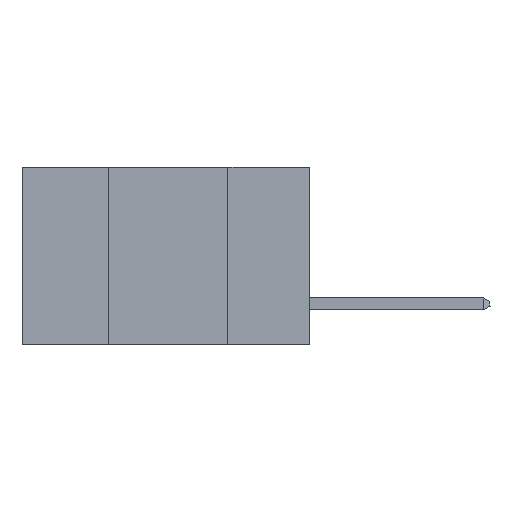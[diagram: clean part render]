
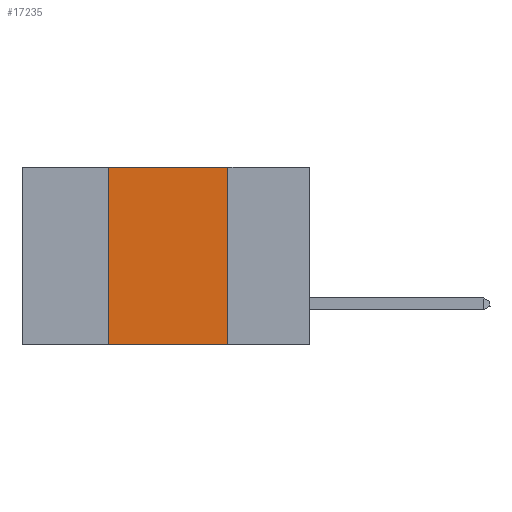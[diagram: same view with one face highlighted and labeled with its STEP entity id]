
A CAD part, left-side view. The second image highlights one B-rep face of the part: STEP entity #17235.
In plain terms, the highlighted planar face has unit normal (-1, 0, 0).
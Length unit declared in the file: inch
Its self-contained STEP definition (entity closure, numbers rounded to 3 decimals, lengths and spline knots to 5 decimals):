
#350 = FACE_OUTER_BOUND ( 'NONE', #6859, .T. ) ;
#2201 = CARTESIAN_POINT ( 'NONE',  ( 0., 0.42, 0. ) ) ;
#5978 = EDGE_CURVE ( 'NONE', #37490, #9699, #15782, .T. ) ;
#6859 = EDGE_LOOP ( 'NONE', ( #36666, #28218, #33068, #27287 ) ) ;
#7327 = LINE ( 'NONE', #34295, #31091 ) ;
#7467 = EDGE_CURVE ( 'NONE', #17618, #29254, #31325, .T. ) ;
#7757 = CARTESIAN_POINT ( 'NONE',  ( 0., 0.6, -0.37 ) ) ;
#9699 = VERTEX_POINT ( 'NONE', #17361 ) ;
#13880 = DIRECTION ( 'NONE',  ( 1., 0., 0. ) ) ;
#14411 = DIRECTION ( 'NONE',  ( 0., -1., 0. ) ) ;
#15782 = LINE ( 'NONE', #23435, #30913 ) ;
#17235 = ADVANCED_FACE ( 'NONE', ( #350 ), #18051, .F. ) ;
#17361 = CARTESIAN_POINT ( 'NONE',  ( 0., 0.17, -0.37 ) ) ;
#17618 = VERTEX_POINT ( 'NONE', #36976 ) ;
#17641 = CARTESIAN_POINT ( 'NONE',  ( 0., 0.42, 0. ) ) ;
#18051 = PLANE ( 'NONE',  #28806 ) ;
#19274 = EDGE_CURVE ( 'NONE', #29254, #37490, #7327, .T. ) ;
#20210 = CARTESIAN_POINT ( 'NONE',  ( 0., 0.6, 0. ) ) ;
#22496 = EDGE_CURVE ( 'NONE', #17618, #9699, #34150, .T. ) ;
#23435 = CARTESIAN_POINT ( 'NONE',  ( 0., 0.17, 0. ) ) ;
#26736 = DIRECTION ( 'NONE',  ( 0., 0., -1. ) ) ;
#27287 = ORIENTED_EDGE ( 'NONE', *, *, #22496, .T. ) ;
#28218 = ORIENTED_EDGE ( 'NONE', *, *, #19274, .F. ) ;
#28806 = AXIS2_PLACEMENT_3D ( 'NONE', #20210, #13880, #30144 ) ;
#29254 = VERTEX_POINT ( 'NONE', #2201 ) ;
#29776 = VECTOR ( 'NONE', #37785, 39.37008 ) ;
#30144 = DIRECTION ( 'NONE',  ( 0., 0., -1. ) ) ;
#30913 = VECTOR ( 'NONE', #26736, 39.37008 ) ;
#31091 = VECTOR ( 'NONE', #14411, 39.37008 ) ;
#31313 = DIRECTION ( 'NONE',  ( 0., -1., 0. ) ) ;
#31325 = LINE ( 'NONE', #17641, #29776 ) ;
#33068 = ORIENTED_EDGE ( 'NONE', *, *, #7467, .F. ) ;
#34150 = LINE ( 'NONE', #7757, #35571 ) ;
#34295 = CARTESIAN_POINT ( 'NONE',  ( 0., 0.6, 0. ) ) ;
#35571 = VECTOR ( 'NONE', #31313, 39.37008 ) ;
#36666 = ORIENTED_EDGE ( 'NONE', *, *, #5978, .F. ) ;
#36976 = CARTESIAN_POINT ( 'NONE',  ( 0., 0.42, -0.37 ) ) ;
#37490 = VERTEX_POINT ( 'NONE', #40091 ) ;
#37785 = DIRECTION ( 'NONE',  ( 0., 0., 1. ) ) ;
#40091 = CARTESIAN_POINT ( 'NONE',  ( 0., 0.17, 0. ) ) ;
